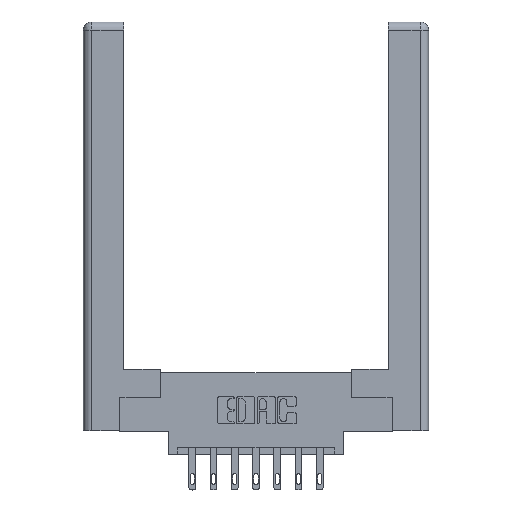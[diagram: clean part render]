
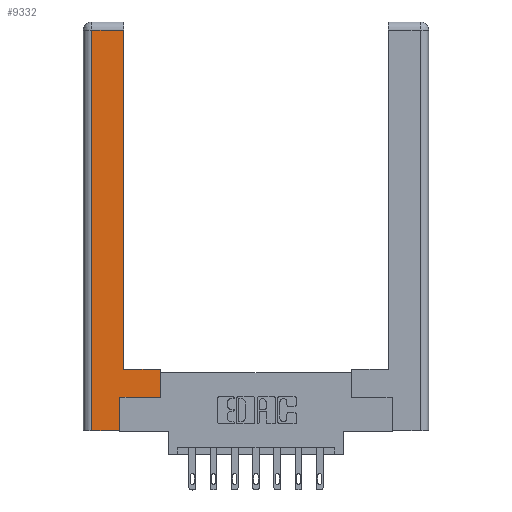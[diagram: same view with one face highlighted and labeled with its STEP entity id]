
A CAD part, top view. The second image highlights one B-rep face of the part: STEP entity #9332.
In plain terms, the highlighted planar face has unit normal (0, 0, 1).
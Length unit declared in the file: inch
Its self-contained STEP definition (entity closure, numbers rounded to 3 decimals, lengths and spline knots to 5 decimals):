
#426 = EDGE_CURVE ( 'NONE', #447, #9009, #5670, .T. ) ;
#436 = CARTESIAN_POINT ( 'NONE',  ( 0.0615, 2.94, 0. ) ) ;
#447 = VERTEX_POINT ( 'NONE', #4490 ) ;
#548 = ORIENTED_EDGE ( 'NONE', *, *, #12586, .T. ) ;
#583 = DIRECTION ( 'NONE',  ( 0., 0., -1. ) ) ;
#732 = VECTOR ( 'NONE', #3499, 39.37008 ) ;
#845 = EDGE_CURVE ( 'NONE', #4489, #8359, #5213, .T. ) ;
#882 = LINE ( 'NONE', #6179, #11001 ) ;
#1435 = CARTESIAN_POINT ( 'NONE',  ( 0.565, 0.45, 0. ) ) ;
#1495 = CARTESIAN_POINT ( 'NONE',  ( 0.265, 0., 0. ) ) ;
#1608 = DIRECTION ( 'NONE',  ( -1., 0., 0. ) ) ;
#2946 = ORIENTED_EDGE ( 'NONE', *, *, #6507, .T. ) ;
#2992 = CARTESIAN_POINT ( 'NONE',  ( 0.265, 0.245, 0. ) ) ;
#3028 = DIRECTION ( 'NONE',  ( 0., 1., 0. ) ) ;
#3051 = CARTESIAN_POINT ( 'NONE',  ( 0.295, 0.45, 0. ) ) ;
#3374 = VECTOR ( 'NONE', #9670, 39.37008 ) ;
#3499 = DIRECTION ( 'NONE',  ( 0., 1., 0. ) ) ;
#3802 = CARTESIAN_POINT ( 'NONE',  ( 0.265, 0., 0. ) ) ;
#3915 = DIRECTION ( 'NONE',  ( -1., 0., 0. ) ) ;
#3997 = CARTESIAN_POINT ( 'NONE',  ( 0.295, 3., 0. ) ) ;
#4254 = CARTESIAN_POINT ( 'NONE',  ( 0.295, 2.94, 0. ) ) ;
#4395 = ORIENTED_EDGE ( 'NONE', *, *, #7900, .T. ) ;
#4489 = VERTEX_POINT ( 'NONE', #3802 ) ;
#4490 = CARTESIAN_POINT ( 'NONE',  ( 0.565, 0.245, 0. ) ) ;
#4769 = LINE ( 'NONE', #11190, #3374 ) ;
#4968 = VECTOR ( 'NONE', #3028, 39.37008 ) ;
#5213 = LINE ( 'NONE', #5605, #12647 ) ;
#5320 = EDGE_CURVE ( 'NONE', #8200, #4489, #10637, .T. ) ;
#5431 = ORIENTED_EDGE ( 'NONE', *, *, #845, .T. ) ;
#5509 = PLANE ( 'NONE',  #12210 ) ;
#5605 = CARTESIAN_POINT ( 'NONE',  ( 0.265, 0.245, 0. ) ) ;
#5647 = ORIENTED_EDGE ( 'NONE', *, *, #11627, .T. ) ;
#5670 = LINE ( 'NONE', #1435, #732 ) ;
#5701 = VERTEX_POINT ( 'NONE', #4254 ) ;
#6076 = DIRECTION ( 'NONE',  ( 0., -1., 0. ) ) ;
#6179 = CARTESIAN_POINT ( 'NONE',  ( 0.565, 0.245, 0. ) ) ;
#6414 = DIRECTION ( 'NONE',  ( 1., 0., 0. ) ) ;
#6475 = CARTESIAN_POINT ( 'NONE',  ( 0.565, 0.45, 0. ) ) ;
#6507 = EDGE_CURVE ( 'NONE', #9009, #7448, #6527, .T. ) ;
#6527 = LINE ( 'NONE', #8613, #11405 ) ;
#7036 = VECTOR ( 'NONE', #6076, 39.37008 ) ;
#7150 = EDGE_LOOP ( 'NONE', ( #4395, #5647, #11105, #9645, #5431, #548, #7431, #2946 ) ) ;
#7431 = ORIENTED_EDGE ( 'NONE', *, *, #426, .T. ) ;
#7448 = VERTEX_POINT ( 'NONE', #3051 ) ;
#7675 = LINE ( 'NONE', #3997, #4968 ) ;
#7714 = CARTESIAN_POINT ( 'NONE',  ( 0.0615, 0., 0. ) ) ;
#7900 = EDGE_CURVE ( 'NONE', #7448, #5701, #7675, .T. ) ;
#7919 = DIRECTION ( 'NONE',  ( 1., 0., 0. ) ) ;
#8200 = VERTEX_POINT ( 'NONE', #7714 ) ;
#8285 = DIRECTION ( 'NONE',  ( 0., 1., 0. ) ) ;
#8359 = VERTEX_POINT ( 'NONE', #2992 ) ;
#8613 = CARTESIAN_POINT ( 'NONE',  ( 0.295, 0.45, 0. ) ) ;
#8905 = CARTESIAN_POINT ( 'NONE',  ( 0.0615, 0., 0. ) ) ;
#9009 = VERTEX_POINT ( 'NONE', #6475 ) ;
#9332 = ADVANCED_FACE ( 'NONE', ( #11013 ), #5509, .F. ) ;
#9385 = VECTOR ( 'NONE', #6414, 39.37008 ) ;
#9455 = VERTEX_POINT ( 'NONE', #436 ) ;
#9584 = LINE ( 'NONE', #8905, #7036 ) ;
#9645 = ORIENTED_EDGE ( 'NONE', *, *, #5320, .T. ) ;
#9670 = DIRECTION ( 'NONE',  ( -1., 0., 0. ) ) ;
#10637 = LINE ( 'NONE', #1495, #9385 ) ;
#11001 = VECTOR ( 'NONE', #7919, 39.37008 ) ;
#11013 = FACE_OUTER_BOUND ( 'NONE', #7150, .T. ) ;
#11105 = ORIENTED_EDGE ( 'NONE', *, *, #11775, .T. ) ;
#11190 = CARTESIAN_POINT ( 'NONE',  ( 0.0615, 2.94, 0. ) ) ;
#11405 = VECTOR ( 'NONE', #3915, 39.37008 ) ;
#11464 = CARTESIAN_POINT ( 'NONE',  ( 0., 0., 0. ) ) ;
#11627 = EDGE_CURVE ( 'NONE', #5701, #9455, #4769, .T. ) ;
#11775 = EDGE_CURVE ( 'NONE', #9455, #8200, #9584, .T. ) ;
#12210 = AXIS2_PLACEMENT_3D ( 'NONE', #11464, #583, #1608 ) ;
#12586 = EDGE_CURVE ( 'NONE', #8359, #447, #882, .T. ) ;
#12647 = VECTOR ( 'NONE', #8285, 39.37008 ) ;
